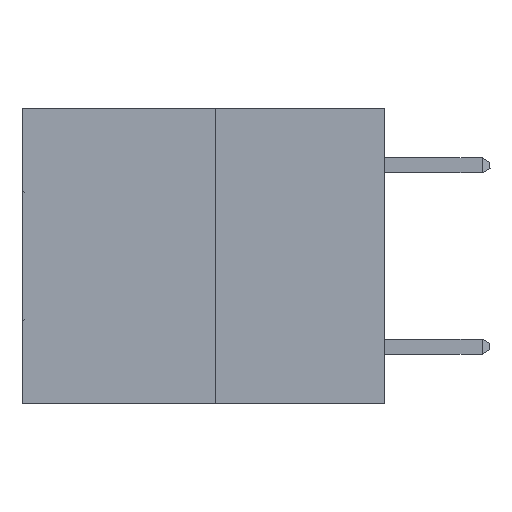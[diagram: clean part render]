
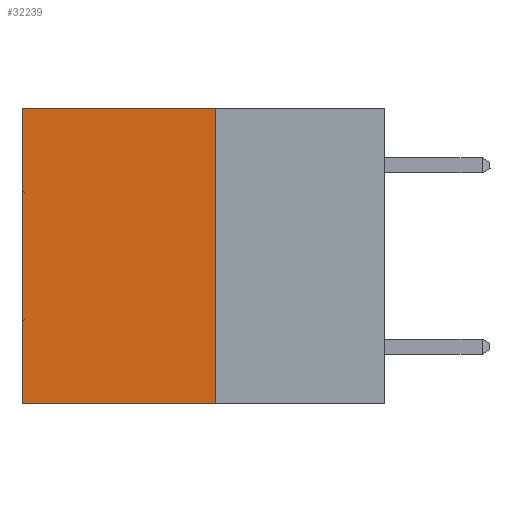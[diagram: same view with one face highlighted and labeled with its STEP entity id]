
A CAD part, left-side view. The second image highlights one B-rep face of the part: STEP entity #32239.
In plain terms, the highlighted planar face has unit normal (-1, 0, 0).
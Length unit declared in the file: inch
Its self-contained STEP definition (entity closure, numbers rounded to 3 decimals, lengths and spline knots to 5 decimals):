
#415 = CARTESIAN_POINT ( 'NONE',  ( 0.3165, 0.28, -0.49 ) ) ;
#657 = DIRECTION ( 'NONE',  ( 0., 0., -1. ) ) ;
#2785 = DIRECTION ( 'NONE',  ( 0., 1., 0. ) ) ;
#3037 = LINE ( 'NONE', #28101, #21419 ) ;
#3118 = AXIS2_PLACEMENT_3D ( 'NONE', #415, #23908, #657 ) ;
#5553 = VERTEX_POINT ( 'NONE', #19923 ) ;
#6639 = EDGE_LOOP ( 'NONE', ( #24802, #7386, #16149, #22718 ) ) ;
#7068 = VECTOR ( 'NONE', #20255, 39.37008 ) ;
#7223 = EDGE_CURVE ( 'NONE', #31658, #20850, #12168, .T. ) ;
#7386 = ORIENTED_EDGE ( 'NONE', *, *, #23198, .F. ) ;
#10674 = FACE_OUTER_BOUND ( 'NONE', #6639, .T. ) ;
#11369 = VECTOR ( 'NONE', #16935, 39.37008 ) ;
#11546 = EDGE_CURVE ( 'NONE', #24007, #31658, #3037, .T. ) ;
#12168 = LINE ( 'NONE', #16616, #11369 ) ;
#12324 = VECTOR ( 'NONE', #2785, 39.37008 ) ;
#14691 = CARTESIAN_POINT ( 'NONE',  ( 0.3165, 0.6, 0. ) ) ;
#16103 = PLANE ( 'NONE',  #3118 ) ;
#16149 = ORIENTED_EDGE ( 'NONE', *, *, #25623, .F. ) ;
#16616 = CARTESIAN_POINT ( 'NONE',  ( 0.3165, 0.6, -0.49 ) ) ;
#16935 = DIRECTION ( 'NONE',  ( 0., 0., -1. ) ) ;
#18008 = LINE ( 'NONE', #31452, #12324 ) ;
#19923 = CARTESIAN_POINT ( 'NONE',  ( 0.3165, 0.28, -0.49 ) ) ;
#20031 = DIRECTION ( 'NONE',  ( 0., 1., 0. ) ) ;
#20255 = DIRECTION ( 'NONE',  ( 0., 0., -1. ) ) ;
#20850 = VERTEX_POINT ( 'NONE', #22078 ) ;
#21419 = VECTOR ( 'NONE', #20031, 39.37008 ) ;
#22078 = CARTESIAN_POINT ( 'NONE',  ( 0.3165, 0.6, -0.49 ) ) ;
#22718 = ORIENTED_EDGE ( 'NONE', *, *, #11546, .T. ) ;
#23198 = EDGE_CURVE ( 'NONE', #5553, #20850, #18008, .T. ) ;
#23908 = DIRECTION ( 'NONE',  ( 1., 0., 0. ) ) ;
#24007 = VERTEX_POINT ( 'NONE', #32642 ) ;
#24802 = ORIENTED_EDGE ( 'NONE', *, *, #7223, .T. ) ;
#25623 = EDGE_CURVE ( 'NONE', #24007, #5553, #31900, .T. ) ;
#28101 = CARTESIAN_POINT ( 'NONE',  ( 0.3165, 0.28, 0. ) ) ;
#31452 = CARTESIAN_POINT ( 'NONE',  ( 0.3165, 0.28, -0.49 ) ) ;
#31658 = VERTEX_POINT ( 'NONE', #14691 ) ;
#31900 = LINE ( 'NONE', #32813, #7068 ) ;
#32239 = ADVANCED_FACE ( 'NONE', ( #10674 ), #16103, .F. ) ;
#32642 = CARTESIAN_POINT ( 'NONE',  ( 0.3165, 0.28, 0. ) ) ;
#32813 = CARTESIAN_POINT ( 'NONE',  ( 0.3165, 0.28, -0.49 ) ) ;
